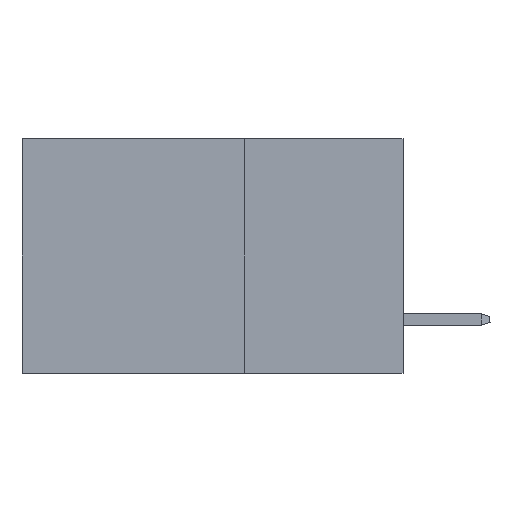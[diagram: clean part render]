
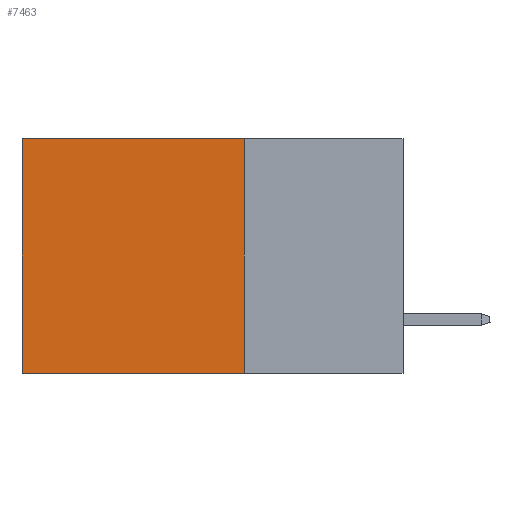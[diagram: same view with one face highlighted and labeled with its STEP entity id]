
A CAD part, left-side view. The second image highlights one B-rep face of the part: STEP entity #7463.
In plain terms, the highlighted planar face has unit normal (-1, 0, 0).
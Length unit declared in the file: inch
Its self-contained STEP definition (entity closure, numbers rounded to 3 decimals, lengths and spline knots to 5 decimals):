
#1017 = CARTESIAN_POINT ( 'NONE',  ( 0.2875, 0.6, 0. ) ) ;
#1079 = FACE_OUTER_BOUND ( 'NONE', #13551, .T. ) ;
#1250 = VECTOR ( 'NONE', #14861, 39.37008 ) ;
#1802 = CARTESIAN_POINT ( 'NONE',  ( 0.2875, 0.6, -0.37 ) ) ;
#4508 = VECTOR ( 'NONE', #24984, 39.37008 ) ;
#7314 = LINE ( 'NONE', #23098, #16801 ) ;
#7463 = ADVANCED_FACE ( 'NONE', ( #1079 ), #16672, .F. ) ;
#9415 = VECTOR ( 'NONE', #18159, 39.37008 ) ;
#9858 = AXIS2_PLACEMENT_3D ( 'NONE', #13938, #26766, #39572 ) ;
#11579 = EDGE_CURVE ( 'NONE', #17634, #30316, #7314, .T. ) ;
#13551 = EDGE_LOOP ( 'NONE', ( #32129, #20893, #35612, #35912 ) ) ;
#13938 = CARTESIAN_POINT ( 'NONE',  ( 0.2875, 0.25, 0. ) ) ;
#14861 = DIRECTION ( 'NONE',  ( 0., 1., 0. ) ) ;
#16672 = PLANE ( 'NONE',  #9858 ) ;
#16801 = VECTOR ( 'NONE', #36103, 39.37008 ) ;
#17634 = VERTEX_POINT ( 'NONE', #29885 ) ;
#18159 = DIRECTION ( 'NONE',  ( 0., 0., -1. ) ) ;
#18360 = LINE ( 'NONE', #37891, #9415 ) ;
#19725 = EDGE_CURVE ( 'NONE', #38185, #30316, #31481, .T. ) ;
#20893 = ORIENTED_EDGE ( 'NONE', *, *, #11579, .F. ) ;
#21990 = LINE ( 'NONE', #28499, #1250 ) ;
#23098 = CARTESIAN_POINT ( 'NONE',  ( 0.2875, 0.25, -0.37 ) ) ;
#24783 = CARTESIAN_POINT ( 'NONE',  ( 0.2875, 0.6, 0. ) ) ;
#24984 = DIRECTION ( 'NONE',  ( 0., 0., -1. ) ) ;
#26766 = DIRECTION ( 'NONE',  ( 1., 0., 0. ) ) ;
#28499 = CARTESIAN_POINT ( 'NONE',  ( 0.2875, 0.25, 0. ) ) ;
#29885 = CARTESIAN_POINT ( 'NONE',  ( 0.2875, 0.25, -0.37 ) ) ;
#29957 = VERTEX_POINT ( 'NONE', #40548 ) ;
#30316 = VERTEX_POINT ( 'NONE', #1802 ) ;
#31481 = LINE ( 'NONE', #24783, #4508 ) ;
#32129 = ORIENTED_EDGE ( 'NONE', *, *, #19725, .T. ) ;
#35612 = ORIENTED_EDGE ( 'NONE', *, *, #39168, .F. ) ;
#35912 = ORIENTED_EDGE ( 'NONE', *, *, #36025, .T. ) ;
#36025 = EDGE_CURVE ( 'NONE', #29957, #38185, #21990, .T. ) ;
#36103 = DIRECTION ( 'NONE',  ( 0., 1., 0. ) ) ;
#37891 = CARTESIAN_POINT ( 'NONE',  ( 0.2875, 0.25, 0. ) ) ;
#38185 = VERTEX_POINT ( 'NONE', #1017 ) ;
#39168 = EDGE_CURVE ( 'NONE', #29957, #17634, #18360, .T. ) ;
#39572 = DIRECTION ( 'NONE',  ( 0., 0., -1. ) ) ;
#40548 = CARTESIAN_POINT ( 'NONE',  ( 0.2875, 0.25, 0. ) ) ;
